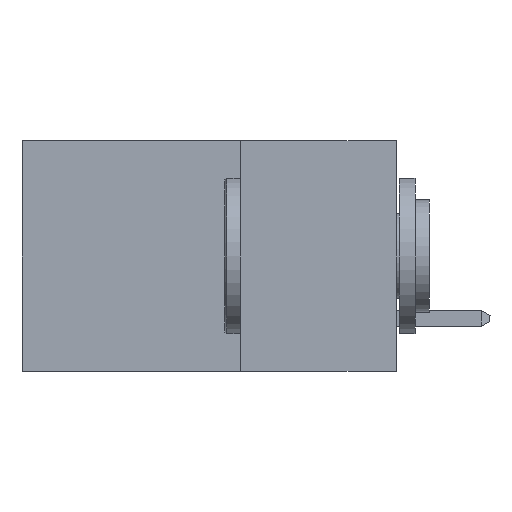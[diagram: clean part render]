
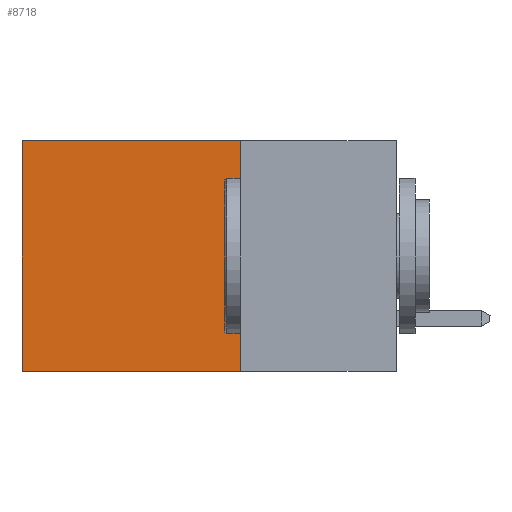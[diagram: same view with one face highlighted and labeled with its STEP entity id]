
A CAD part, left-side view. The second image highlights one B-rep face of the part: STEP entity #8718.
In plain terms, the highlighted planar face has unit normal (-1, 0, 0).
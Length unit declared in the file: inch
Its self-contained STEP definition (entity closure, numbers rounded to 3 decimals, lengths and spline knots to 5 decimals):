
#235 = AXIS2_PLACEMENT_3D ( 'NONE', #1093, #7559, #2804 ) ;
#671 = VERTEX_POINT ( 'NONE', #10460 ) ;
#979 = CARTESIAN_POINT ( 'NONE',  ( 0.2615, 0.25, -0.37 ) ) ;
#1093 = CARTESIAN_POINT ( 'NONE',  ( 0.2615, 0.25, -0.37 ) ) ;
#1222 = ORIENTED_EDGE ( 'NONE', *, *, #8620, .F. ) ;
#1812 = VECTOR ( 'NONE', #3695, 39.37008 ) ;
#2181 = LINE ( 'NONE', #9963, #8070 ) ;
#2804 = DIRECTION ( 'NONE',  ( 0., 0., -1. ) ) ;
#3354 = LINE ( 'NONE', #979, #7314 ) ;
#3437 = EDGE_CURVE ( 'NONE', #4953, #671, #7492, .T. ) ;
#3693 = CARTESIAN_POINT ( 'NONE',  ( 0.2615, 0.6, -0.37 ) ) ;
#3695 = DIRECTION ( 'NONE',  ( 0., 0., -1. ) ) ;
#4006 = CARTESIAN_POINT ( 'NONE',  ( 0.2615, 0.6, 0. ) ) ;
#4510 = FACE_OUTER_BOUND ( 'NONE', #6439, .T. ) ;
#4935 = VECTOR ( 'NONE', #5477, 39.37008 ) ;
#4953 = VERTEX_POINT ( 'NONE', #7840 ) ;
#5296 = VERTEX_POINT ( 'NONE', #4006 ) ;
#5314 = CARTESIAN_POINT ( 'NONE',  ( 0.2615, 0.25, -0.37 ) ) ;
#5477 = DIRECTION ( 'NONE',  ( 0., 0., -1. ) ) ;
#5760 = EDGE_CURVE ( 'NONE', #4953, #5296, #2181, .T. ) ;
#6439 = EDGE_LOOP ( 'NONE', ( #9054, #1222, #7664, #8176 ) ) ;
#6773 = PLANE ( 'NONE',  #235 ) ;
#7007 = EDGE_CURVE ( 'NONE', #5296, #9890, #7966, .T. ) ;
#7314 = VECTOR ( 'NONE', #8230, 39.37008 ) ;
#7492 = LINE ( 'NONE', #5314, #4935 ) ;
#7559 = DIRECTION ( 'NONE',  ( 1., 0., 0. ) ) ;
#7664 = ORIENTED_EDGE ( 'NONE', *, *, #3437, .F. ) ;
#7840 = CARTESIAN_POINT ( 'NONE',  ( 0.2615, 0.25, 0. ) ) ;
#7966 = LINE ( 'NONE', #3693, #1812 ) ;
#8070 = VECTOR ( 'NONE', #9944, 39.37008 ) ;
#8176 = ORIENTED_EDGE ( 'NONE', *, *, #5760, .T. ) ;
#8230 = DIRECTION ( 'NONE',  ( 0., 1., 0. ) ) ;
#8620 = EDGE_CURVE ( 'NONE', #671, #9890, #3354, .T. ) ;
#8718 = ADVANCED_FACE ( 'NONE', ( #4510 ), #6773, .F. ) ;
#9054 = ORIENTED_EDGE ( 'NONE', *, *, #7007, .T. ) ;
#9121 = CARTESIAN_POINT ( 'NONE',  ( 0.2615, 0.6, -0.37 ) ) ;
#9890 = VERTEX_POINT ( 'NONE', #9121 ) ;
#9944 = DIRECTION ( 'NONE',  ( 0., 1., 0. ) ) ;
#9963 = CARTESIAN_POINT ( 'NONE',  ( 0.2615, 0.25, 0. ) ) ;
#10460 = CARTESIAN_POINT ( 'NONE',  ( 0.2615, 0.25, -0.37 ) ) ;
